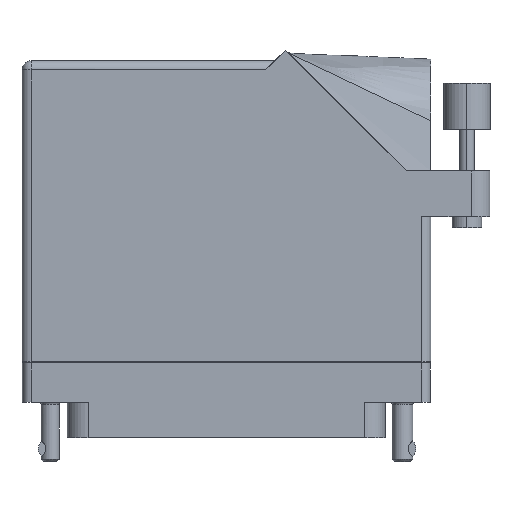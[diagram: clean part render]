
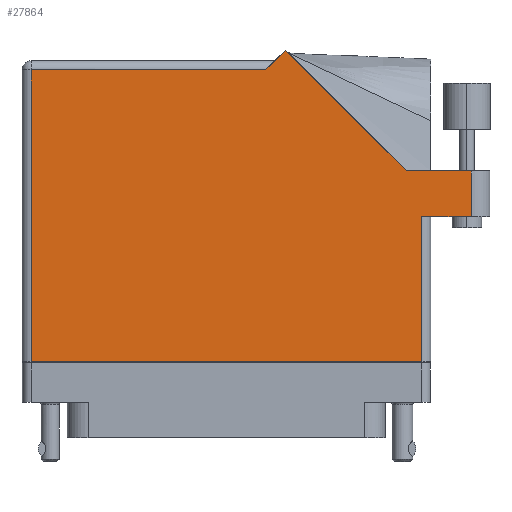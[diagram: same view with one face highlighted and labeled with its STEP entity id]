
A CAD part, front view. The second image highlights one B-rep face of the part: STEP entity #27864.
In plain terms, the highlighted face is planar.
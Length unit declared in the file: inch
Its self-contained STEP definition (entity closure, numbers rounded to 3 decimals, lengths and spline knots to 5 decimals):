
#368 = EDGE_CURVE ( 'NONE', #54040, #13787, #89941, .T. ) ;
#2824 = ORIENTED_EDGE ( 'NONE', *, *, #79882, .T. ) ;
#7444 = VECTOR ( 'NONE', #43947, 39.37008 ) ;
#7573 = LINE ( 'NONE', #77834, #50638 ) ;
#8204 = CARTESIAN_POINT ( 'NONE',  ( 1.6525, 1.187, 0.765 ) ) ;
#8244 = EDGE_CURVE ( 'NONE', #26616, #96118, #7573, .T. ) ;
#8969 = ORIENTED_EDGE ( 'NONE', *, *, #40596, .T. ) ;
#9495 = VECTOR ( 'NONE', #12440, 39.37008 ) ;
#10891 = CARTESIAN_POINT ( 'NONE',  ( -1.3775, -0.1, 0.765 ) ) ;
#12140 = CARTESIAN_POINT ( 'NONE',  ( -1.3155, 1.868, 0.765 ) ) ;
#12440 = DIRECTION ( 'NONE',  ( -0.707, -0.707, 0. ) ) ;
#13162 = CARTESIAN_POINT ( 'NONE',  ( 1.3155, 0.88, 0.765 ) ) ;
#13705 = DIRECTION ( 'NONE',  ( 0., 1., 0. ) ) ;
#13787 = VERTEX_POINT ( 'NONE', #43695 ) ;
#15588 = ORIENTED_EDGE ( 'NONE', *, *, #82647, .T. ) ;
#16524 = LINE ( 'NONE', #64233, #9495 ) ;
#20202 = VECTOR ( 'NONE', #70805, 39.37008 ) ;
#20261 = CARTESIAN_POINT ( 'NONE',  ( 1.3155, 0.88, 0.765 ) ) ;
#25116 = DIRECTION ( 'NONE',  ( 0., -1., 0. ) ) ;
#25151 = ORIENTED_EDGE ( 'NONE', *, *, #32257, .T. ) ;
#25309 = CARTESIAN_POINT ( 'NONE',  ( -1.3155, -0.1, 0.765 ) ) ;
#26616 = VERTEX_POINT ( 'NONE', #12140 ) ;
#26632 = VECTOR ( 'NONE', #52540, 39.37008 ) ;
#27272 = LINE ( 'NONE', #88576, #7444 ) ;
#27722 = EDGE_CURVE ( 'NONE', #96118, #84717, #59743, .T. ) ;
#27864 = ADVANCED_FACE ( 'NONE', ( #56346 ), #36852, .F. ) ;
#28606 = VERTEX_POINT ( 'NONE', #35240 ) ;
#29459 = CARTESIAN_POINT ( 'NONE',  ( 1.7775, 1.187, 0.765 ) ) ;
#30952 = CARTESIAN_POINT ( 'NONE',  ( 1.6525, 0.88, 0.765 ) ) ;
#32257 = EDGE_CURVE ( 'NONE', #90137, #49028, #43735, .T. ) ;
#33307 = CARTESIAN_POINT ( 'NONE',  ( -1.3775, 1.868, 0.765 ) ) ;
#34039 = LINE ( 'NONE', #20261, #79446 ) ;
#34201 = EDGE_CURVE ( 'NONE', #84717, #90137, #34039, .T. ) ;
#35240 = CARTESIAN_POINT ( 'NONE',  ( 0.2655, 1.868, 0.765 ) ) ;
#36852 = PLANE ( 'NONE',  #47265 ) ;
#37311 = CARTESIAN_POINT ( 'NONE',  ( 1.3155, -0.1, 0.765 ) ) ;
#40596 = EDGE_CURVE ( 'NONE', #49028, #71539, #27272, .T. ) ;
#41701 = LINE ( 'NONE', #29459, #26632 ) ;
#41825 = ORIENTED_EDGE ( 'NONE', *, *, #27722, .T. ) ;
#43695 = CARTESIAN_POINT ( 'NONE',  ( 0.39821, 2.00071, 0.765 ) ) ;
#43735 = LINE ( 'NONE', #65417, #75238 ) ;
#43947 = DIRECTION ( 'NONE',  ( 0., 1., 0. ) ) ;
#44328 = DIRECTION ( 'NONE',  ( -1., 0., 0. ) ) ;
#47265 = AXIS2_PLACEMENT_3D ( 'NONE', #89915, #88973, #44328 ) ;
#49028 = VERTEX_POINT ( 'NONE', #30952 ) ;
#50415 = DIRECTION ( 'NONE',  ( 1., 0., 0. ) ) ;
#50638 = VECTOR ( 'NONE', #25116, 39.37008 ) ;
#52540 = DIRECTION ( 'NONE',  ( -1., 0., 0. ) ) ;
#53322 = CARTESIAN_POINT ( 'NONE',  ( 1.21192, 1.187, 0.765 ) ) ;
#54040 = VERTEX_POINT ( 'NONE', #53322 ) ;
#56346 = FACE_OUTER_BOUND ( 'NONE', #83694, .T. ) ;
#59396 = ORIENTED_EDGE ( 'NONE', *, *, #34201, .T. ) ;
#59743 = LINE ( 'NONE', #10891, #20202 ) ;
#64233 = CARTESIAN_POINT ( 'NONE',  ( 0.3275, 1.93, 0.765 ) ) ;
#64766 = DIRECTION ( 'NONE',  ( -0.707, 0.707, 0. ) ) ;
#65417 = CARTESIAN_POINT ( 'NONE',  ( 1.3775, 0.88, 0.765 ) ) ;
#65493 = VECTOR ( 'NONE', #64766, 39.37008 ) ;
#65734 = ORIENTED_EDGE ( 'NONE', *, *, #8244, .T. ) ;
#67846 = ORIENTED_EDGE ( 'NONE', *, *, #368, .T. ) ;
#70114 = DIRECTION ( 'NONE',  ( -1., 0., 0. ) ) ;
#70805 = DIRECTION ( 'NONE',  ( 1., 0., 0. ) ) ;
#71539 = VERTEX_POINT ( 'NONE', #8204 ) ;
#75238 = VECTOR ( 'NONE', #50415, 39.37008 ) ;
#77834 = CARTESIAN_POINT ( 'NONE',  ( -1.3155, -0.1, 0.765 ) ) ;
#78930 = VECTOR ( 'NONE', #70114, 39.37008 ) ;
#79402 = CARTESIAN_POINT ( 'NONE',  ( 1.21192, 1.187, 0.765 ) ) ;
#79446 = VECTOR ( 'NONE', #13705, 39.37008 ) ;
#79882 = EDGE_CURVE ( 'NONE', #13787, #28606, #16524, .T. ) ;
#81282 = LINE ( 'NONE', #33307, #78930 ) ;
#82647 = EDGE_CURVE ( 'NONE', #28606, #26616, #81282, .T. ) ;
#82797 = ORIENTED_EDGE ( 'NONE', *, *, #96538, .T. ) ;
#83694 = EDGE_LOOP ( 'NONE', ( #25151, #8969, #82797, #67846, #2824, #15588, #65734, #41825, #59396 ) ) ;
#84717 = VERTEX_POINT ( 'NONE', #37311 ) ;
#88576 = CARTESIAN_POINT ( 'NONE',  ( 1.6525, 1.187, 0.765 ) ) ;
#88973 = DIRECTION ( 'NONE',  ( 0., 0., -1. ) ) ;
#89915 = CARTESIAN_POINT ( 'NONE',  ( -1.3775, 1.93, 0.765 ) ) ;
#89941 = LINE ( 'NONE', #79402, #65493 ) ;
#90137 = VERTEX_POINT ( 'NONE', #13162 ) ;
#96118 = VERTEX_POINT ( 'NONE', #25309 ) ;
#96538 = EDGE_CURVE ( 'NONE', #71539, #54040, #41701, .T. ) ;
